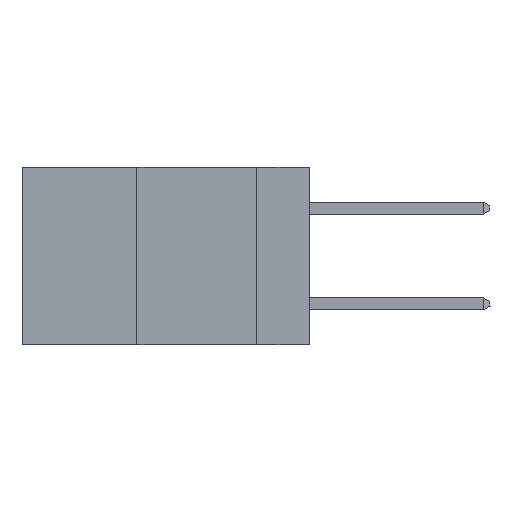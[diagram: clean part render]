
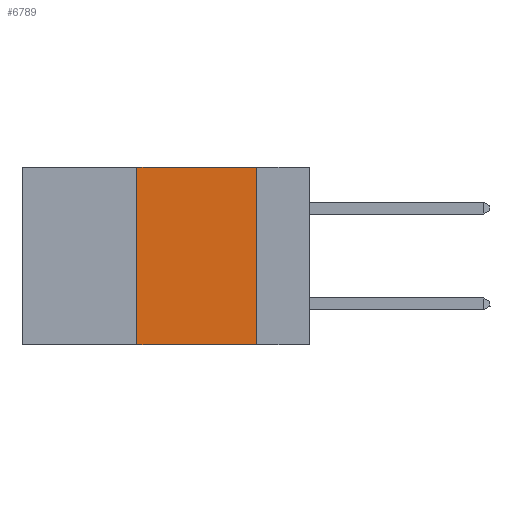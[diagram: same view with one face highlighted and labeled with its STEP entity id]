
A CAD part, left-side view. The second image highlights one B-rep face of the part: STEP entity #6789.
In plain terms, the highlighted planar face has unit normal (-1, 0, 0).
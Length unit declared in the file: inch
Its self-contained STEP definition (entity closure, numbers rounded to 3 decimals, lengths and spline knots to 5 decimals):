
#405 = ORIENTED_EDGE ( 'NONE', *, *, #3516, .T. ) ;
#1242 = CARTESIAN_POINT ( 'NONE',  ( 0., 0.6, 0. ) ) ;
#1556 = AXIS2_PLACEMENT_3D ( 'NONE', #1242, #12323, #14062 ) ;
#1744 = VECTOR ( 'NONE', #5349, 39.37008 ) ;
#3156 = EDGE_CURVE ( 'NONE', #12331, #6095, #5389, .T. ) ;
#3274 = EDGE_LOOP ( 'NONE', ( #4462, #14581, #13224, #405 ) ) ;
#3516 = EDGE_CURVE ( 'NONE', #14836, #6095, #4853, .T. ) ;
#4136 = VECTOR ( 'NONE', #16447, 39.37008 ) ;
#4430 = CARTESIAN_POINT ( 'NONE',  ( 0., 0.36, 0. ) ) ;
#4462 = ORIENTED_EDGE ( 'NONE', *, *, #3156, .F. ) ;
#4853 = LINE ( 'NONE', #5172, #4136 ) ;
#5172 = CARTESIAN_POINT ( 'NONE',  ( 0., 0.6, -0.37 ) ) ;
#5287 = CARTESIAN_POINT ( 'NONE',  ( 0., 0.36, 0. ) ) ;
#5349 = DIRECTION ( 'NONE',  ( 0., -1., 0. ) ) ;
#5389 = LINE ( 'NONE', #10556, #19676 ) ;
#6095 = VERTEX_POINT ( 'NONE', #7002 ) ;
#6245 = CARTESIAN_POINT ( 'NONE',  ( 0., 0.11, 0. ) ) ;
#6789 = ADVANCED_FACE ( 'NONE', ( #20442 ), #17277, .F. ) ;
#7002 = CARTESIAN_POINT ( 'NONE',  ( 0., 0.11, -0.37 ) ) ;
#7033 = CARTESIAN_POINT ( 'NONE',  ( 0., 0.6, 0. ) ) ;
#7825 = CARTESIAN_POINT ( 'NONE',  ( 0., 0.36, -0.37 ) ) ;
#8704 = VECTOR ( 'NONE', #9382, 39.37008 ) ;
#8928 = DIRECTION ( 'NONE',  ( 0., 0., -1. ) ) ;
#9382 = DIRECTION ( 'NONE',  ( 0., 0., 1. ) ) ;
#10507 = VERTEX_POINT ( 'NONE', #5287 ) ;
#10556 = CARTESIAN_POINT ( 'NONE',  ( 0., 0.11, 0. ) ) ;
#10691 = EDGE_CURVE ( 'NONE', #10507, #12331, #12019, .T. ) ;
#12019 = LINE ( 'NONE', #7033, #1744 ) ;
#12273 = EDGE_CURVE ( 'NONE', #14836, #10507, #17271, .T. ) ;
#12323 = DIRECTION ( 'NONE',  ( 1., 0., 0. ) ) ;
#12331 = VERTEX_POINT ( 'NONE', #6245 ) ;
#13224 = ORIENTED_EDGE ( 'NONE', *, *, #12273, .F. ) ;
#14062 = DIRECTION ( 'NONE',  ( 0., 0., -1. ) ) ;
#14581 = ORIENTED_EDGE ( 'NONE', *, *, #10691, .F. ) ;
#14836 = VERTEX_POINT ( 'NONE', #7825 ) ;
#16447 = DIRECTION ( 'NONE',  ( 0., -1., 0. ) ) ;
#17271 = LINE ( 'NONE', #4430, #8704 ) ;
#17277 = PLANE ( 'NONE',  #1556 ) ;
#19676 = VECTOR ( 'NONE', #8928, 39.37008 ) ;
#20442 = FACE_OUTER_BOUND ( 'NONE', #3274, .T. ) ;
